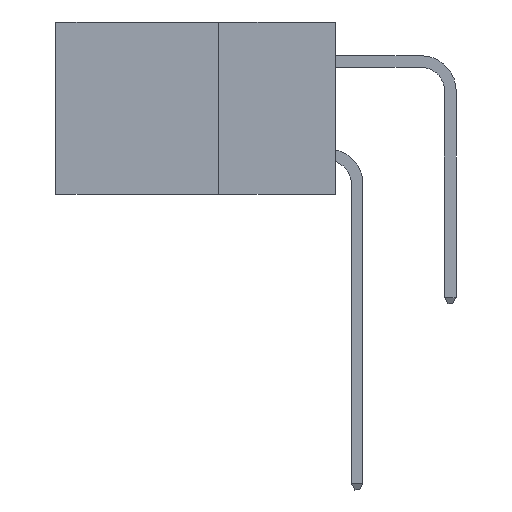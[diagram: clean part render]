
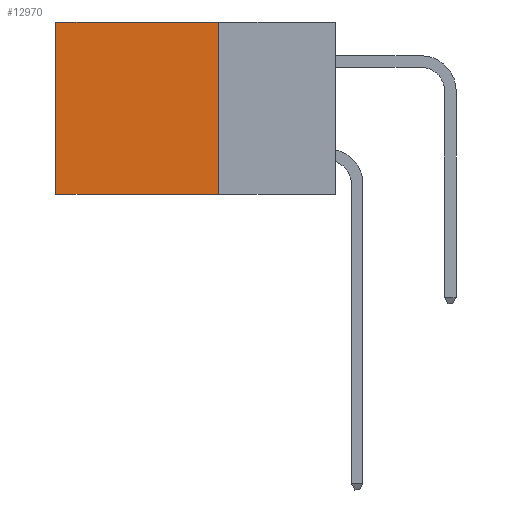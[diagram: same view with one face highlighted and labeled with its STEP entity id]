
A CAD part, left-side view. The second image highlights one B-rep face of the part: STEP entity #12970.
In plain terms, the highlighted planar face has unit normal (-1, 0, 0).
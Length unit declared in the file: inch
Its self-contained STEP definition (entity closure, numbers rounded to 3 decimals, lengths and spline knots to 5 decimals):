
#139 = EDGE_CURVE ( 'NONE', #16524, #2926, #1953, .T. ) ;
#716 = VECTOR ( 'NONE', #20771, 39.37008 ) ;
#1025 = CARTESIAN_POINT ( 'NONE',  ( 0.2875, 0.25, 0. ) ) ;
#1953 = LINE ( 'NONE', #12796, #716 ) ;
#2926 = VERTEX_POINT ( 'NONE', #25013 ) ;
#3275 = VECTOR ( 'NONE', #17879, 39.37008 ) ;
#3832 = LINE ( 'NONE', #22131, #5661 ) ;
#5217 = LINE ( 'NONE', #20376, #18470 ) ;
#5661 = VECTOR ( 'NONE', #10381, 39.37008 ) ;
#5898 = ORIENTED_EDGE ( 'NONE', *, *, #139, .T. ) ;
#5964 = CARTESIAN_POINT ( 'NONE',  ( 0.2875, 0.25, -0.37 ) ) ;
#6318 = AXIS2_PLACEMENT_3D ( 'NONE', #1025, #20593, #24690 ) ;
#7860 = ORIENTED_EDGE ( 'NONE', *, *, #20957, .F. ) ;
#10381 = DIRECTION ( 'NONE',  ( 0., 0., -1. ) ) ;
#12017 = ORIENTED_EDGE ( 'NONE', *, *, #13581, .T. ) ;
#12416 = CARTESIAN_POINT ( 'NONE',  ( 0.2875, 0.25, -0.37 ) ) ;
#12649 = DIRECTION ( 'NONE',  ( 0., 0., -1. ) ) ;
#12796 = CARTESIAN_POINT ( 'NONE',  ( 0.2875, 0.25, 0. ) ) ;
#12970 = ADVANCED_FACE ( 'NONE', ( #15430 ), #16829, .F. ) ;
#13581 = EDGE_CURVE ( 'NONE', #2926, #20245, #5217, .T. ) ;
#15430 = FACE_OUTER_BOUND ( 'NONE', #19500, .T. ) ;
#16524 = VERTEX_POINT ( 'NONE', #19866 ) ;
#16829 = PLANE ( 'NONE',  #6318 ) ;
#17733 = ORIENTED_EDGE ( 'NONE', *, *, #21042, .F. ) ;
#17879 = DIRECTION ( 'NONE',  ( 0., 1., 0. ) ) ;
#18470 = VECTOR ( 'NONE', #12649, 39.37008 ) ;
#19201 = CARTESIAN_POINT ( 'NONE',  ( 0.2875, 0.6, -0.37 ) ) ;
#19500 = EDGE_LOOP ( 'NONE', ( #12017, #7860, #17733, #5898 ) ) ;
#19866 = CARTESIAN_POINT ( 'NONE',  ( 0.2875, 0.25, 0. ) ) ;
#20245 = VERTEX_POINT ( 'NONE', #19201 ) ;
#20376 = CARTESIAN_POINT ( 'NONE',  ( 0.2875, 0.6, 0. ) ) ;
#20593 = DIRECTION ( 'NONE',  ( 1., 0., 0. ) ) ;
#20771 = DIRECTION ( 'NONE',  ( 0., 1., 0. ) ) ;
#20957 = EDGE_CURVE ( 'NONE', #21681, #20245, #24758, .T. ) ;
#21042 = EDGE_CURVE ( 'NONE', #16524, #21681, #3832, .T. ) ;
#21681 = VERTEX_POINT ( 'NONE', #12416 ) ;
#22131 = CARTESIAN_POINT ( 'NONE',  ( 0.2875, 0.25, 0. ) ) ;
#24690 = DIRECTION ( 'NONE',  ( 0., 0., -1. ) ) ;
#24758 = LINE ( 'NONE', #5964, #3275 ) ;
#25013 = CARTESIAN_POINT ( 'NONE',  ( 0.2875, 0.6, 0. ) ) ;
